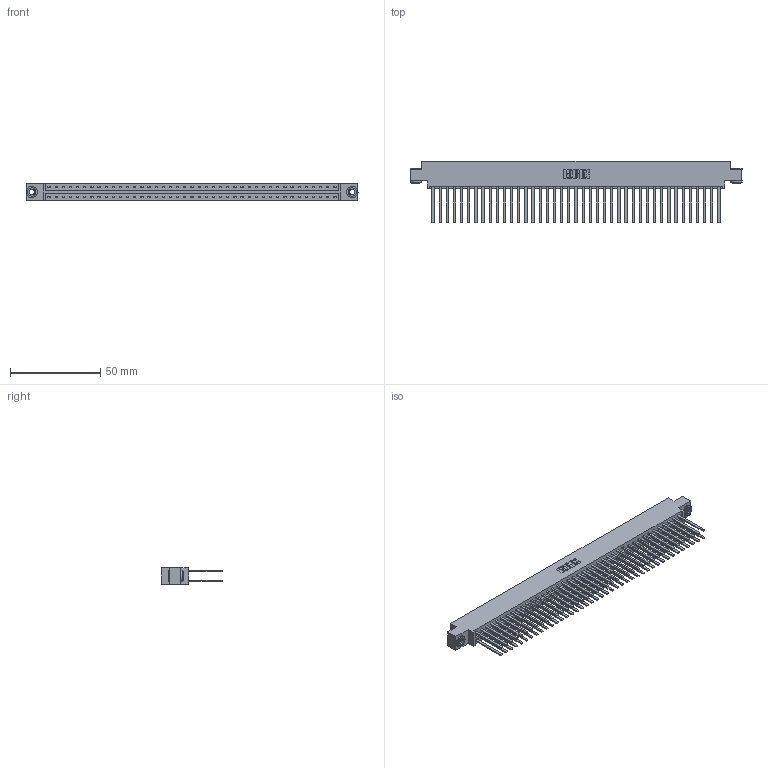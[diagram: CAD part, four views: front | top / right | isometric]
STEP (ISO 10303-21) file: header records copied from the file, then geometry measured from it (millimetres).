
FILE_DESCRIPTION (( 'STEP AP203' ), '1' );
FILE_NAME ('333-082-544-803.STEP', '2018-08-05T03:20:15', ( '' ), ( '' ), 'SwSTEP 2.0', 'SolidWorks 2016', '' );
FILE_SCHEMA (( 'CONFIG_CONTROL_DESIGN' ));
Length unit declared in the file: inch
Products named in the file (4): 333 Part_Offset - .156 Dia - TH; 345-292-001_345-293-144; 345-250-002_345-250-002-102; 333-082-544-803
Assembly tree (85 placements, depth 2):
  333-082-544-803
    333 Part_Offset - .156 Dia - TH
    345-292-001_345-293-144  x82
    345-250-002_345-250-002-102  x2
Bounding box: 184 x 34.3 x 9.4 mm (x, y, z)
Volume: 19716.8 mm3; surface area: 27442.2 mm2
Topology: 85 solids, 85 shells, 3928 faces, 11633 edges, 7642 vertices
Faces by surface type: plane 2708, cylinder 1212, cone 8
Entity records: 27104 total; most frequent: CARTESIAN_POINT 4469, ORIENTED_EDGE 4398, DIRECTION 3849, EDGE_CURVE 2199, LINE 2051, VECTOR 2051, VERTEX_POINT 1462, AXIS2_PLACEMENT_3D 899
